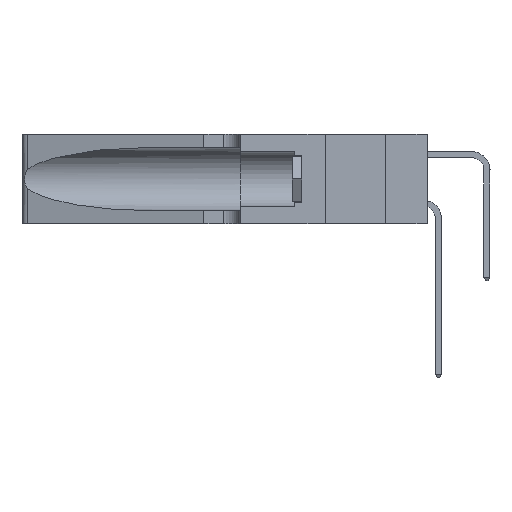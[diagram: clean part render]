
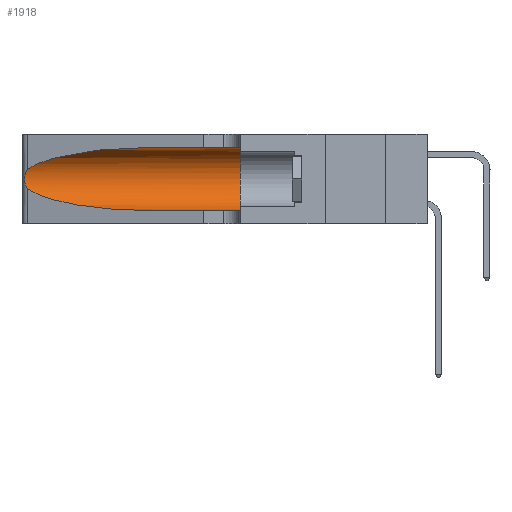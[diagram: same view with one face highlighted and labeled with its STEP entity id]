
A CAD part, left-side view. The second image highlights one B-rep face of the part: STEP entity #1918.
In plain terms, the highlighted cylindrical face has radius 3.308 mm (diameter 6.617 mm), a partial arc.
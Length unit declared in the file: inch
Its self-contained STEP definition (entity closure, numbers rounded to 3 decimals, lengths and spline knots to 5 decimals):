
#1160 =( BOUNDED_CURVE ( )  B_SPLINE_CURVE ( 3, ( #1840, #3872, #17521, #5934 ),
 .UNSPECIFIED., .F., .F. ) 
 B_SPLINE_CURVE_WITH_KNOTS ( ( 4, 4 ),
 ( 3.44316, 4.71239 ),
 .UNSPECIFIED. ) 
 CURVE ( )  GEOMETRIC_REPRESENTATION_ITEM ( )  RATIONAL_B_SPLINE_CURVE ( ( 1., 0.87, 0.87, 1. ) ) 
 REPRESENTATION_ITEM ( '' )  );
#1502 = B_SPLINE_CURVE_WITH_KNOTS ( 'NONE', 3,
 ( #5937, #17525, #13768, #1927, #15678, #3980, #17607, #6025, #19514, #8050, #21416, #10045, #23298, #11971 ),
 .UNSPECIFIED., .F., .F.,
 ( 4, 2, 2, 2, 2, 2, 4 ),
 ( 0., 0.00027, 0.00053, 0.00107, 0.0016, 0.00187, 0.00214 ),
 .UNSPECIFIED. ) ;
#1840 = CARTESIAN_POINT ( 'NONE',  ( 0.25487, 1.22718, 0.14631 ) ) ;
#1918 = ADVANCED_FACE ( 'NONE', ( #3061 ), #18024, .F. ) ;
#1927 = CARTESIAN_POINT ( 'NONE',  ( 0.25787, 1.23484, 0.2124 ) ) ;
#2812 = VERTEX_POINT ( 'NONE', #11254 ) ;
#3061 = FACE_OUTER_BOUND ( 'NONE', #7958, .T. ) ;
#3143 =( BOUNDED_CURVE ( )  B_SPLINE_CURVE ( 3, ( #20977, #19081, #7590, #9575 ),
 .UNSPECIFIED., .F., .F. ) 
 B_SPLINE_CURVE_WITH_KNOTS ( ( 4, 4 ),
 ( 1.5708, 2.84003 ),
 .UNSPECIFIED. ) 
 CURVE ( )  GEOMETRIC_REPRESENTATION_ITEM ( )  RATIONAL_B_SPLINE_CURVE ( ( 1., 0.87, 0.87, 1. ) ) 
 REPRESENTATION_ITEM ( '' )  );
#3184 = CARTESIAN_POINT ( 'NONE',  ( 0.1305, 1.61858, 0.05475 ) ) ;
#3224 = CARTESIAN_POINT ( 'NONE',  ( 0.1305, 0.72297, 0.05475 ) ) ;
#3872 = CARTESIAN_POINT ( 'NONE',  ( 0.2373, 1.15595, 0.08982 ) ) ;
#3980 = CARTESIAN_POINT ( 'NONE',  ( 0.26018, 1.23835, 0.19895 ) ) ;
#4078 = VECTOR ( 'NONE', #20667, 39.37008 ) ;
#4567 = ORIENTED_EDGE ( 'NONE', *, *, #22924, .T. ) ;
#4739 = CARTESIAN_POINT ( 'NONE',  ( 0.25487, 1.22718, 0.22369 ) ) ;
#5085 = CIRCLE ( 'NONE', #14415, 0.13025 ) ;
#5934 = CARTESIAN_POINT ( 'NONE',  ( 0.1305, 0.72297, 0.05475 ) ) ;
#5937 = CARTESIAN_POINT ( 'NONE',  ( 0.25487, 1.22718, 0.22369 ) ) ;
#6025 = CARTESIAN_POINT ( 'NONE',  ( 0.26075, 1.23896, 0.178 ) ) ;
#6796 = VECTOR ( 'NONE', #18316, 39.37008 ) ;
#7372 = DIRECTION ( 'NONE',  ( 0., 1., 0. ) ) ;
#7590 = CARTESIAN_POINT ( 'NONE',  ( 0.2373, 1.15595, 0.28018 ) ) ;
#7958 = EDGE_LOOP ( 'NONE', ( #9109, #14428, #4567, #12175, #11609, #8056 ) ) ;
#8047 = LINE ( 'NONE', #20119, #6796 ) ;
#8050 = CARTESIAN_POINT ( 'NONE',  ( 0.25856, 1.23593, 0.16098 ) ) ;
#8056 = ORIENTED_EDGE ( 'NONE', *, *, #13568, .F. ) ;
#8468 = CARTESIAN_POINT ( 'NONE',  ( 0.1305, 0.35, 0.05475 ) ) ;
#9109 = ORIENTED_EDGE ( 'NONE', *, *, #15077, .T. ) ;
#9575 = CARTESIAN_POINT ( 'NONE',  ( 0.25487, 1.22718, 0.22369 ) ) ;
#10045 = CARTESIAN_POINT ( 'NONE',  ( 0.25639, 1.23186, 0.15144 ) ) ;
#10862 = EDGE_CURVE ( 'NONE', #20136, #24995, #19571, .T. ) ;
#11218 = CARTESIAN_POINT ( 'NONE',  ( 0.1305, 0.35, 0.31525 ) ) ;
#11254 = CARTESIAN_POINT ( 'NONE',  ( 0.25487, 1.22718, 0.14631 ) ) ;
#11609 = ORIENTED_EDGE ( 'NONE', *, *, #22235, .F. ) ;
#11971 = CARTESIAN_POINT ( 'NONE',  ( 0.25487, 1.22718, 0.14631 ) ) ;
#12175 = ORIENTED_EDGE ( 'NONE', *, *, #10862, .T. ) ;
#13568 = EDGE_CURVE ( 'NONE', #15544, #22720, #8047, .T. ) ;
#13768 = CARTESIAN_POINT ( 'NONE',  ( 0.25639, 1.23184, 0.21858 ) ) ;
#14415 = AXIS2_PLACEMENT_3D ( 'NONE', #18886, #7372, #20773 ) ;
#14428 = ORIENTED_EDGE ( 'NONE', *, *, #20994, .T. ) ;
#15077 = EDGE_CURVE ( 'NONE', #15544, #23896, #3143, .T. ) ;
#15544 = VERTEX_POINT ( 'NONE', #24664 ) ;
#15678 = CARTESIAN_POINT ( 'NONE',  ( 0.25854, 1.2359, 0.20912 ) ) ;
#17521 = CARTESIAN_POINT ( 'NONE',  ( 0.18966, 0.96281, 0.05475 ) ) ;
#17525 = CARTESIAN_POINT ( 'NONE',  ( 0.25555, 1.22994, 0.2215 ) ) ;
#17607 = CARTESIAN_POINT ( 'NONE',  ( 0.26075, 1.23896, 0.19203 ) ) ;
#18024 = CYLINDRICAL_SURFACE ( 'NONE', #21472, 0.13025 ) ;
#18316 = DIRECTION ( 'NONE',  ( 0., -1., 0. ) ) ;
#18886 = CARTESIAN_POINT ( 'NONE',  ( 0.1305, 0.35, 0.185 ) ) ;
#19081 = CARTESIAN_POINT ( 'NONE',  ( 0.18966, 0.96281, 0.31525 ) ) ;
#19514 = CARTESIAN_POINT ( 'NONE',  ( 0.26017, 1.23833, 0.17102 ) ) ;
#19518 = DIRECTION ( 'NONE',  ( 0., -1., 0. ) ) ;
#19571 = LINE ( 'NONE', #3184, #4078 ) ;
#20119 = CARTESIAN_POINT ( 'NONE',  ( 0.1305, 1.61858, 0.31525 ) ) ;
#20136 = VERTEX_POINT ( 'NONE', #3224 ) ;
#20667 = DIRECTION ( 'NONE',  ( 0., -1., 0. ) ) ;
#20773 = DIRECTION ( 'NONE',  ( 0., 0., 1. ) ) ;
#20977 = CARTESIAN_POINT ( 'NONE',  ( 0.1305, 0.72297, 0.31525 ) ) ;
#20994 = EDGE_CURVE ( 'NONE', #23896, #2812, #1502, .T. ) ;
#21416 = CARTESIAN_POINT ( 'NONE',  ( 0.25789, 1.23486, 0.15765 ) ) ;
#21472 = AXIS2_PLACEMENT_3D ( 'NONE', #23457, #19518, #23383 ) ;
#22235 = EDGE_CURVE ( 'NONE', #22720, #24995, #5085, .T. ) ;
#22720 = VERTEX_POINT ( 'NONE', #11218 ) ;
#22924 = EDGE_CURVE ( 'NONE', #2812, #20136, #1160, .T. ) ;
#23298 = CARTESIAN_POINT ( 'NONE',  ( 0.25555, 1.22993, 0.14849 ) ) ;
#23383 = DIRECTION ( 'NONE',  ( 0., 0., -1. ) ) ;
#23457 = CARTESIAN_POINT ( 'NONE',  ( 0.1305, 1.61858, 0.185 ) ) ;
#23896 = VERTEX_POINT ( 'NONE', #4739 ) ;
#24664 = CARTESIAN_POINT ( 'NONE',  ( 0.1305, 0.72297, 0.31525 ) ) ;
#24995 = VERTEX_POINT ( 'NONE', #8468 ) ;
